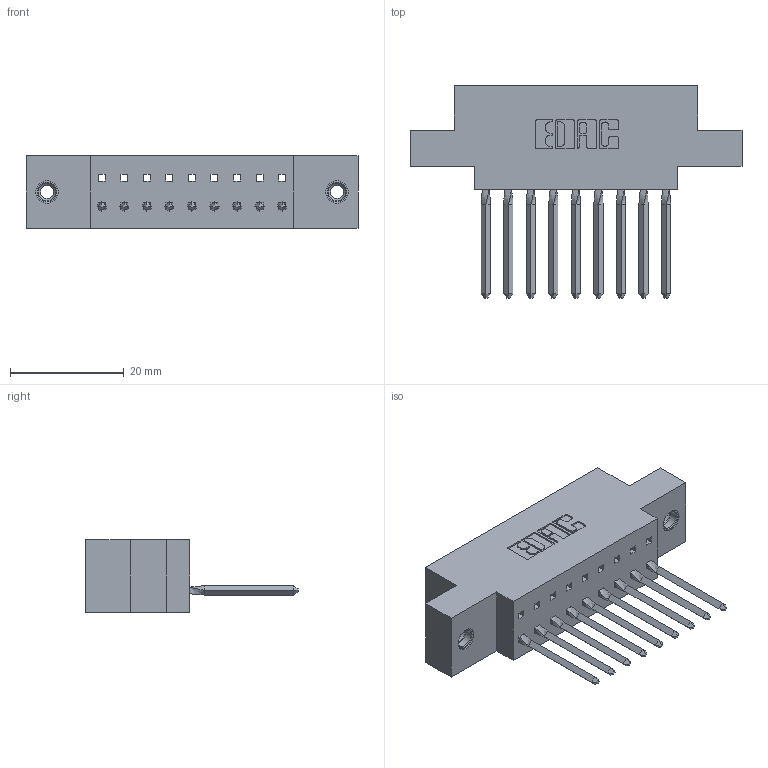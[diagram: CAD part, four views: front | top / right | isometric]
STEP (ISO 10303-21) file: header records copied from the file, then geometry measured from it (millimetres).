
FILE_DESCRIPTION (( 'STEP AP203' ), '1' );
FILE_NAME ('317-009-542-678.STEP', '2020-02-27T13:18:36', ( '' ), ( '' ), 'SwSTEP 2.0', 'SolidWorks 2016', '' );
FILE_SCHEMA (( 'CONFIG_CONTROL_DESIGN' ));
Length unit declared in the file: inch
Products named in the file (4): 317-009-542-678; 345-250-001_345-250-003-102; 317 Part_.156 Dia - TI; 317-290-003_542
Assembly tree (12 placements, depth 2):
  317-009-542-678
    317 Part_.156 Dia - TI
    317-290-003_542  x9
    345-250-001_345-250-003-102  x2
Bounding box: 58.37 x 37.34 x 12.7 mm (x, y, z)
Volume: 8132.5 mm3; surface area: 9204.4 mm2
Topology: 12 solids, 12 shells, 837 faces, 2364 edges, 1526 vertices
Faces by surface type: plane 666, cylinder 119, bspline 36, cone 12, torus 4
Entity records: 17528 total; most frequent: CARTESIAN_POINT 3315, ORIENTED_EDGE 2980, DIRECTION 2586, EDGE_CURVE 1490, VECTOR 1300, LINE 1300, VERTEX_POINT 984, AXIS2_PLACEMENT_3D 643
